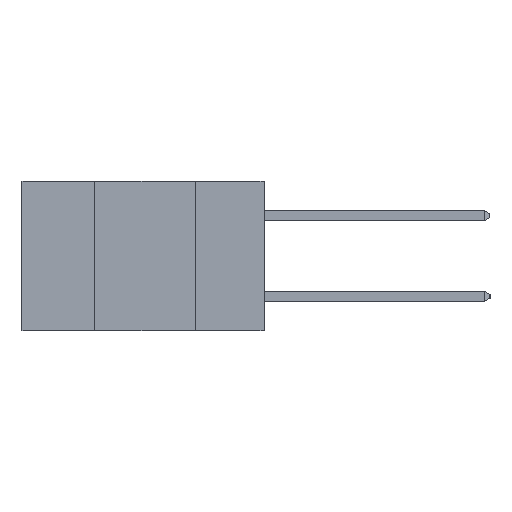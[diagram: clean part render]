
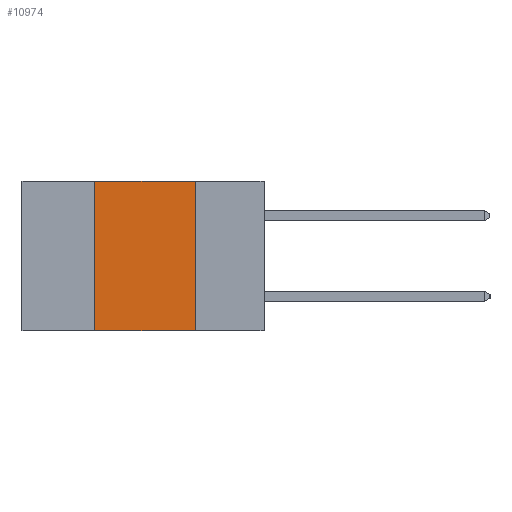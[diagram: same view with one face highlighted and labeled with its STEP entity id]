
A CAD part, left-side view. The second image highlights one B-rep face of the part: STEP entity #10974.
In plain terms, the highlighted planar face has unit normal (-1, 0, 0).
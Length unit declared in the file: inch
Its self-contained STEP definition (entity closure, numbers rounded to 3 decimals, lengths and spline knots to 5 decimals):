
#2 = LINE ( 'NONE', #10141, #19763 ) ;
#28 = CARTESIAN_POINT ( 'NONE',  ( 0., 0.6, -0.37 ) ) ;
#1487 = LINE ( 'NONE', #28, #23052 ) ;
#2138 = DIRECTION ( 'NONE',  ( 0., -1., 0. ) ) ;
#2534 = CARTESIAN_POINT ( 'NONE',  ( 0., 0.17, -0.37 ) ) ;
#2717 = CARTESIAN_POINT ( 'NONE',  ( 0., 0.6, 0. ) ) ;
#2804 = CARTESIAN_POINT ( 'NONE',  ( 0., 0.42, 0. ) ) ;
#3171 = DIRECTION ( 'NONE',  ( 0., -1., 0. ) ) ;
#3478 = CARTESIAN_POINT ( 'NONE',  ( 0., 0.42, -0.37 ) ) ;
#3538 = CARTESIAN_POINT ( 'NONE',  ( 0., 0.17, 0. ) ) ;
#3547 = CARTESIAN_POINT ( 'NONE',  ( 0., 0.6, 0. ) ) ;
#4096 = EDGE_CURVE ( 'NONE', #25764, #17318, #14179, .T. ) ;
#4749 = PLANE ( 'NONE',  #17340 ) ;
#4754 = ORIENTED_EDGE ( 'NONE', *, *, #6469, .F. ) ;
#5935 = LINE ( 'NONE', #12367, #20805 ) ;
#6365 = DIRECTION ( 'NONE',  ( 0., 0., 1. ) ) ;
#6469 = EDGE_CURVE ( 'NONE', #17318, #24249, #2, .T. ) ;
#8909 = DIRECTION ( 'NONE',  ( 0., 0., -1. ) ) ;
#8962 = ORIENTED_EDGE ( 'NONE', *, *, #4096, .F. ) ;
#10081 = EDGE_CURVE ( 'NONE', #11909, #24249, #1487, .T. ) ;
#10141 = CARTESIAN_POINT ( 'NONE',  ( 0., 0.17, -0.37 ) ) ;
#10974 = ADVANCED_FACE ( 'NONE', ( #18554 ), #4749, .F. ) ;
#11909 = VERTEX_POINT ( 'NONE', #3478 ) ;
#12176 = DIRECTION ( 'NONE',  ( 0., 0., -1. ) ) ;
#12367 = CARTESIAN_POINT ( 'NONE',  ( 0., 0.42, -0.37 ) ) ;
#12395 = ORIENTED_EDGE ( 'NONE', *, *, #10081, .T. ) ;
#14179 = LINE ( 'NONE', #3547, #24192 ) ;
#16385 = EDGE_CURVE ( 'NONE', #11909, #25764, #5935, .T. ) ;
#17318 = VERTEX_POINT ( 'NONE', #3538 ) ;
#17340 = AXIS2_PLACEMENT_3D ( 'NONE', #2717, #20997, #8909 ) ;
#18554 = FACE_OUTER_BOUND ( 'NONE', #22730, .T. ) ;
#19763 = VECTOR ( 'NONE', #12176, 39.37008 ) ;
#20805 = VECTOR ( 'NONE', #6365, 39.37008 ) ;
#20997 = DIRECTION ( 'NONE',  ( 1., 0., 0. ) ) ;
#22730 = EDGE_LOOP ( 'NONE', ( #4754, #8962, #23730, #12395 ) ) ;
#23052 = VECTOR ( 'NONE', #2138, 39.37008 ) ;
#23730 = ORIENTED_EDGE ( 'NONE', *, *, #16385, .F. ) ;
#24192 = VECTOR ( 'NONE', #3171, 39.37008 ) ;
#24249 = VERTEX_POINT ( 'NONE', #2534 ) ;
#25764 = VERTEX_POINT ( 'NONE', #2804 ) ;
